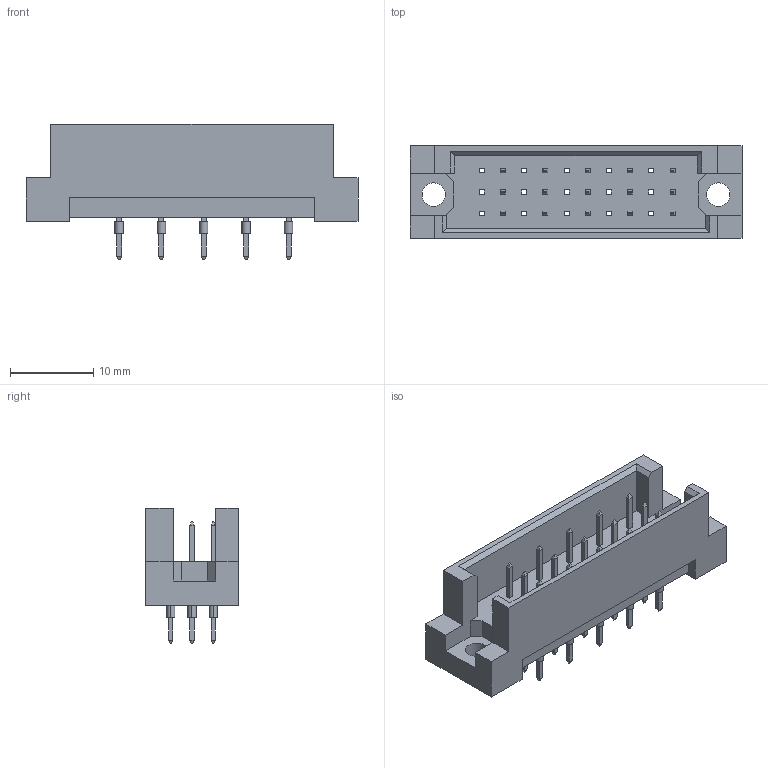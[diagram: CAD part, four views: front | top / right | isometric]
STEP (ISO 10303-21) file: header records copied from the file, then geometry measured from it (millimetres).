
FILE_DESCRIPTION (( 'STEP AP203' ), '1' );
FILE_NAME ('493-115-270-321.STEP', '2019-11-11T18:38:00', ( '' ), ( '' ), 'SwSTEP 2.0', 'SolidWorks 2020', '' );
FILE_SCHEMA (( 'CONFIG_CONTROL_DESIGN' ));
Length unit declared in the file: millimetre
Products named in the file (3): 493 Part_30; 493-115-270-321; 493-290_70
Assembly tree (16 placements, depth 2):
  493-115-270-321
    493 Part_30
    493-290_70  x15
Bounding box: 39.8 x 11.1 x 16.2 mm (x, y, z)
Volume: 2448 mm3; surface area: 3249.5 mm2
Topology: 16 solids, 16 shells, 502 faces, 1196 edges, 756 vertices
Faces by surface type: plane 468, cylinder 34
Entity records: 7053 total; most frequent: CARTESIAN_POINT 1129, ORIENTED_EDGE 1104, DIRECTION 990, EDGE_CURVE 552, VECTOR 540, LINE 540, VERTEX_POINT 364, EDGE_LOOP 260
